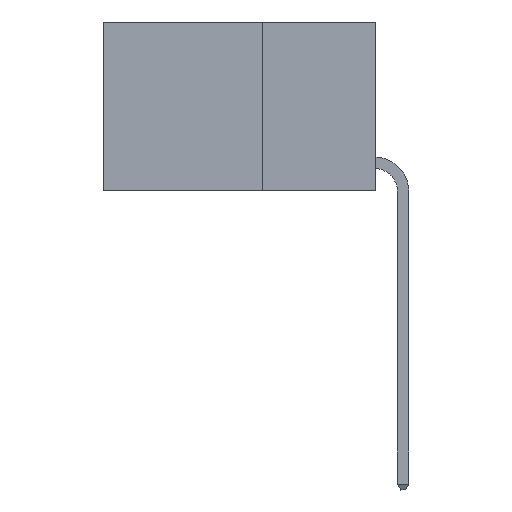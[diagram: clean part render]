
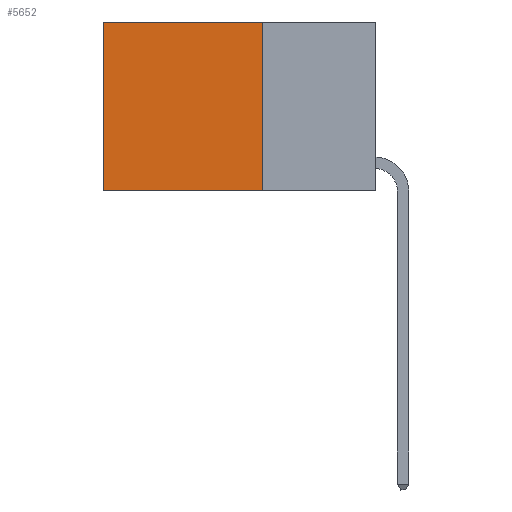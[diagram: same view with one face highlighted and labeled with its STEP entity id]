
A CAD part, left-side view. The second image highlights one B-rep face of the part: STEP entity #5652.
In plain terms, the highlighted planar face has unit normal (-1, 0, 0).
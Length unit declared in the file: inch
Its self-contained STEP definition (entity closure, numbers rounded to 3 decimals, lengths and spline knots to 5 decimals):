
#418 = CARTESIAN_POINT ( 'NONE',  ( 0.2625, 0.25, -0.37 ) ) ;
#566 = DIRECTION ( 'NONE',  ( 0., 0., -1. ) ) ;
#928 = VERTEX_POINT ( 'NONE', #8808 ) ;
#932 = EDGE_CURVE ( 'NONE', #7138, #7364, #3269, .T. ) ;
#1267 = VECTOR ( 'NONE', #4376, 39.37008 ) ;
#1283 = LINE ( 'NONE', #418, #4345 ) ;
#1336 = DIRECTION ( 'NONE',  ( 0., 1., 0. ) ) ;
#1543 = ORIENTED_EDGE ( 'NONE', *, *, #8276, .T. ) ;
#1557 = AXIS2_PLACEMENT_3D ( 'NONE', #9082, #3836, #10807 ) ;
#1617 = VECTOR ( 'NONE', #8143, 39.37008 ) ;
#1915 = PLANE ( 'NONE',  #1557 ) ;
#2376 = CARTESIAN_POINT ( 'NONE',  ( 0.2625, 0.25, 0. ) ) ;
#2907 = EDGE_CURVE ( 'NONE', #8539, #928, #8543, .T. ) ;
#3269 = LINE ( 'NONE', #2376, #1267 ) ;
#3413 = ORIENTED_EDGE ( 'NONE', *, *, #2907, .T. ) ;
#3820 = EDGE_LOOP ( 'NONE', ( #3413, #8951, #8934, #1543 ) ) ;
#3836 = DIRECTION ( 'NONE',  ( 1., 0., 0. ) ) ;
#4345 = VECTOR ( 'NONE', #1336, 39.37008 ) ;
#4376 = DIRECTION ( 'NONE',  ( 0., 0., -1. ) ) ;
#4834 = CARTESIAN_POINT ( 'NONE',  ( 0.2625, 0.25, 0. ) ) ;
#5241 = CARTESIAN_POINT ( 'NONE',  ( 0.2625, 0.6, 0. ) ) ;
#5547 = FACE_OUTER_BOUND ( 'NONE', #3820, .T. ) ;
#5652 = ADVANCED_FACE ( 'NONE', ( #5547 ), #1915, .F. ) ;
#6516 = CARTESIAN_POINT ( 'NONE',  ( 0.2625, 0.6, 0. ) ) ;
#6991 = EDGE_CURVE ( 'NONE', #7364, #928, #1283, .T. ) ;
#7138 = VERTEX_POINT ( 'NONE', #4834 ) ;
#7364 = VERTEX_POINT ( 'NONE', #8258 ) ;
#8143 = DIRECTION ( 'NONE',  ( 0., 1., 0. ) ) ;
#8258 = CARTESIAN_POINT ( 'NONE',  ( 0.2625, 0.25, -0.37 ) ) ;
#8276 = EDGE_CURVE ( 'NONE', #7138, #8539, #9747, .T. ) ;
#8539 = VERTEX_POINT ( 'NONE', #5241 ) ;
#8543 = LINE ( 'NONE', #6516, #10248 ) ;
#8808 = CARTESIAN_POINT ( 'NONE',  ( 0.2625, 0.6, -0.37 ) ) ;
#8860 = CARTESIAN_POINT ( 'NONE',  ( 0.2625, 0.25, 0. ) ) ;
#8934 = ORIENTED_EDGE ( 'NONE', *, *, #932, .F. ) ;
#8951 = ORIENTED_EDGE ( 'NONE', *, *, #6991, .F. ) ;
#9082 = CARTESIAN_POINT ( 'NONE',  ( 0.2625, 0.25, 0. ) ) ;
#9747 = LINE ( 'NONE', #8860, #1617 ) ;
#10248 = VECTOR ( 'NONE', #566, 39.37008 ) ;
#10807 = DIRECTION ( 'NONE',  ( 0., 0., -1. ) ) ;
